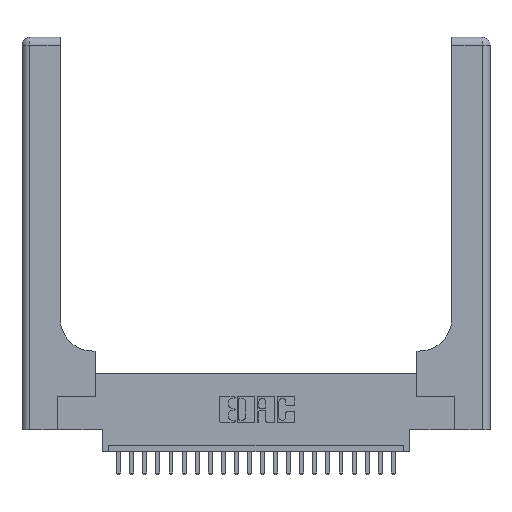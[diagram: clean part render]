
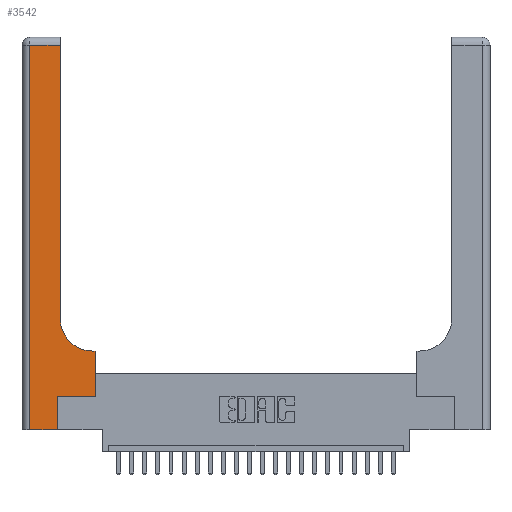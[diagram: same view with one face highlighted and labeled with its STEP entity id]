
A CAD part, top view. The second image highlights one B-rep face of the part: STEP entity #3542.
In plain terms, the highlighted planar face has unit normal (0, 0, 1).
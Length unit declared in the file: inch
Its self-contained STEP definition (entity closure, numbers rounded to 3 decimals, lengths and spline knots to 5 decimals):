
#106 = CARTESIAN_POINT ( 'NONE',  ( 0.06, 0., 0.37 ) ) ;
#574 = ORIENTED_EDGE ( 'NONE', *, *, #21006, .T. ) ;
#705 = VERTEX_POINT ( 'NONE', #20910 ) ;
#1006 = CARTESIAN_POINT ( 'NONE',  ( 0.06, 3., 0.37 ) ) ;
#1854 = CARTESIAN_POINT ( 'NONE',  ( 0.5585, 0.25, 0.37 ) ) ;
#2251 = FACE_OUTER_BOUND ( 'NONE', #6407, .T. ) ;
#2431 = CARTESIAN_POINT ( 'NONE',  ( 0.2915, 3., 0.37 ) ) ;
#2604 = VERTEX_POINT ( 'NONE', #24142 ) ;
#3472 = CARTESIAN_POINT ( 'NONE',  ( 0.269, 0., 0.37 ) ) ;
#3542 = ADVANCED_FACE ( 'NONE', ( #2251 ), #10062, .F. ) ;
#4000 = AXIS2_PLACEMENT_3D ( 'NONE', #19626, #8604, #4777 ) ;
#4147 = CARTESIAN_POINT ( 'NONE',  ( 0.2915, 2.94, 0.37 ) ) ;
#4164 = DIRECTION ( 'NONE',  ( 1., 0., 0. ) ) ;
#4777 = DIRECTION ( 'NONE',  ( -1., 0., 0. ) ) ;
#5124 = LINE ( 'NONE', #1854, #24514 ) ;
#5448 = VERTEX_POINT ( 'NONE', #7702 ) ;
#5477 = VERTEX_POINT ( 'NONE', #106 ) ;
#5529 = DIRECTION ( 'NONE',  ( 0., 1., 0. ) ) ;
#5695 = LINE ( 'NONE', #20603, #5990 ) ;
#5795 = EDGE_CURVE ( 'NONE', #5448, #11352, #5124, .T. ) ;
#5902 = EDGE_CURVE ( 'NONE', #19375, #705, #18573, .T. ) ;
#5990 = VECTOR ( 'NONE', #9182, 39.37008 ) ;
#6407 = EDGE_LOOP ( 'NONE', ( #574, #19957, #23384, #18747, #15676, #11690, #8546, #12484, #10183 ) ) ;
#6722 = DIRECTION ( 'NONE',  ( -1., 0., 0. ) ) ;
#6731 = LINE ( 'NONE', #18943, #16933 ) ;
#7018 = EDGE_CURVE ( 'NONE', #11352, #19375, #16193, .T. ) ;
#7616 = DIRECTION ( 'NONE',  ( -1., 0., 0. ) ) ;
#7702 = CARTESIAN_POINT ( 'NONE',  ( 0.5585, 0.25, 0.37 ) ) ;
#8012 = CARTESIAN_POINT ( 'NONE',  ( 0.269, 0.25, 0.37 ) ) ;
#8531 = VECTOR ( 'NONE', #7616, 39.37008 ) ;
#8546 = ORIENTED_EDGE ( 'NONE', *, *, #5795, .T. ) ;
#8604 = DIRECTION ( 'NONE',  ( 0., 0., -1. ) ) ;
#9182 = DIRECTION ( 'NONE',  ( 1., 0., 0. ) ) ;
#10062 = PLANE ( 'NONE',  #4000 ) ;
#10183 = ORIENTED_EDGE ( 'NONE', *, *, #5902, .T. ) ;
#10255 = EDGE_CURVE ( 'NONE', #2604, #5477, #19864, .T. ) ;
#10502 = CARTESIAN_POINT ( 'NONE',  ( 0.5585, 0.6, 0.37 ) ) ;
#10871 = CARTESIAN_POINT ( 'NONE',  ( 0.5415, 0.6, 0.37 ) ) ;
#11104 = VECTOR ( 'NONE', #6722, 39.37008 ) ;
#11352 = VERTEX_POINT ( 'NONE', #10502 ) ;
#11554 = DIRECTION ( 'NONE',  ( 0., 0., -1. ) ) ;
#11558 = LINE ( 'NONE', #2431, #21075 ) ;
#11690 = ORIENTED_EDGE ( 'NONE', *, *, #20858, .T. ) ;
#12231 = AXIS2_PLACEMENT_3D ( 'NONE', #21196, #11554, #4164 ) ;
#12366 = CARTESIAN_POINT ( 'NONE',  ( 0.2915, 0.6, 0.37 ) ) ;
#12455 = VECTOR ( 'NONE', #14413, 39.37008 ) ;
#12484 = ORIENTED_EDGE ( 'NONE', *, *, #7018, .T. ) ;
#13059 = EDGE_CURVE ( 'NONE', #14610, #24186, #20823, .T. ) ;
#13735 = DIRECTION ( 'NONE',  ( 0., 1., 0. ) ) ;
#14019 = VECTOR ( 'NONE', #5529, 39.37008 ) ;
#14237 = EDGE_CURVE ( 'NONE', #23686, #2604, #24067, .T. ) ;
#14413 = DIRECTION ( 'NONE',  ( 0., -1., 0. ) ) ;
#14610 = VERTEX_POINT ( 'NONE', #3472 ) ;
#14856 = CARTESIAN_POINT ( 'NONE',  ( 0.269, 0., 0.37 ) ) ;
#15398 = DIRECTION ( 'NONE',  ( 1., 0., 0. ) ) ;
#15676 = ORIENTED_EDGE ( 'NONE', *, *, #13059, .T. ) ;
#16193 = LINE ( 'NONE', #12366, #11104 ) ;
#16933 = VECTOR ( 'NONE', #15398, 39.37008 ) ;
#18365 = DIRECTION ( 'NONE',  ( 0., 1., 0. ) ) ;
#18573 = CIRCLE ( 'NONE', #12231, 0.25 ) ;
#18747 = ORIENTED_EDGE ( 'NONE', *, *, #23423, .T. ) ;
#18943 = CARTESIAN_POINT ( 'NONE',  ( 0.269, 0.25, 0.37 ) ) ;
#19035 = CARTESIAN_POINT ( 'NONE',  ( 0., 2.94, 0.37 ) ) ;
#19375 = VERTEX_POINT ( 'NONE', #10871 ) ;
#19626 = CARTESIAN_POINT ( 'NONE',  ( 0., 3., 0.37 ) ) ;
#19864 = LINE ( 'NONE', #1006, #12455 ) ;
#19957 = ORIENTED_EDGE ( 'NONE', *, *, #14237, .T. ) ;
#20603 = CARTESIAN_POINT ( 'NONE',  ( 0., 0., 0.37 ) ) ;
#20823 = LINE ( 'NONE', #14856, #14019 ) ;
#20858 = EDGE_CURVE ( 'NONE', #24186, #5448, #6731, .T. ) ;
#20910 = CARTESIAN_POINT ( 'NONE',  ( 0.2915, 0.85, 0.37 ) ) ;
#21006 = EDGE_CURVE ( 'NONE', #705, #23686, #11558, .T. ) ;
#21075 = VECTOR ( 'NONE', #13735, 39.37008 ) ;
#21196 = CARTESIAN_POINT ( 'NONE',  ( 0.5415, 0.85, 0.37 ) ) ;
#23384 = ORIENTED_EDGE ( 'NONE', *, *, #10255, .T. ) ;
#23423 = EDGE_CURVE ( 'NONE', #5477, #14610, #5695, .T. ) ;
#23686 = VERTEX_POINT ( 'NONE', #4147 ) ;
#24067 = LINE ( 'NONE', #19035, #8531 ) ;
#24142 = CARTESIAN_POINT ( 'NONE',  ( 0.06, 2.94, 0.37 ) ) ;
#24186 = VERTEX_POINT ( 'NONE', #8012 ) ;
#24514 = VECTOR ( 'NONE', #18365, 39.37008 ) ;
